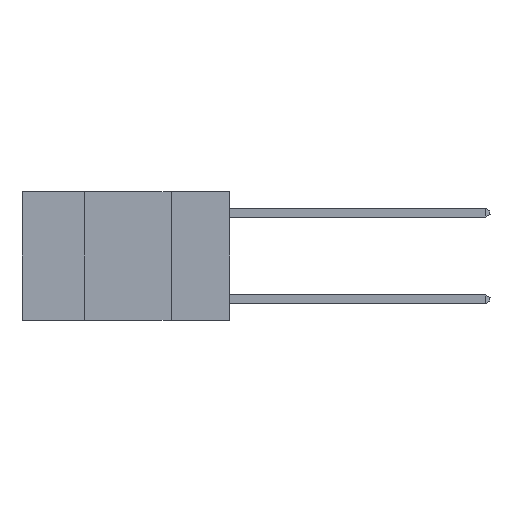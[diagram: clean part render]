
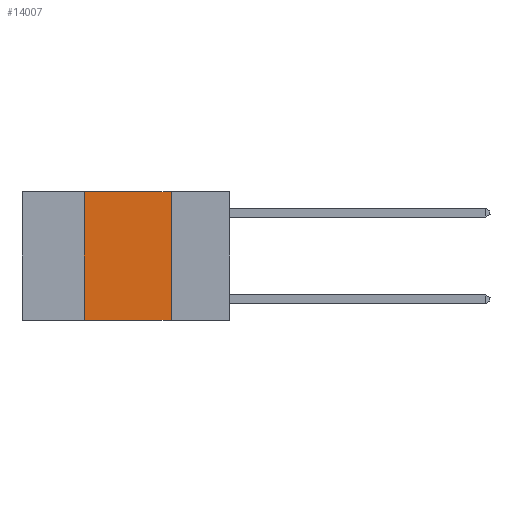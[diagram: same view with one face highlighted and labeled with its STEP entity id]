
A CAD part, left-side view. The second image highlights one B-rep face of the part: STEP entity #14007.
In plain terms, the highlighted planar face has unit normal (-1, 0, 0).
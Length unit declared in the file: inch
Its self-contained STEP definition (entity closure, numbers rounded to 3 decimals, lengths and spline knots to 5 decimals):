
#234 = FACE_OUTER_BOUND ( 'NONE', #3559, .T. ) ;
#333 = CARTESIAN_POINT ( 'NONE',  ( 0., 0.17, 0. ) ) ;
#428 = EDGE_CURVE ( 'NONE', #11161, #1083, #12738, .T. ) ;
#554 = ORIENTED_EDGE ( 'NONE', *, *, #428, .F. ) ;
#1083 = VERTEX_POINT ( 'NONE', #3482 ) ;
#1178 = DIRECTION ( 'NONE',  ( 0., 0., 1. ) ) ;
#1195 = VERTEX_POINT ( 'NONE', #333 ) ;
#1783 = DIRECTION ( 'NONE',  ( 0., -1., 0. ) ) ;
#2016 = VERTEX_POINT ( 'NONE', #6250 ) ;
#2127 = ORIENTED_EDGE ( 'NONE', *, *, #10634, .F. ) ;
#2310 = DIRECTION ( 'NONE',  ( 0., 0., -1. ) ) ;
#2327 = ORIENTED_EDGE ( 'NONE', *, *, #3384, .T. ) ;
#2596 = LINE ( 'NONE', #10588, #4030 ) ;
#3384 = EDGE_CURVE ( 'NONE', #11161, #2016, #12032, .T. ) ;
#3482 = CARTESIAN_POINT ( 'NONE',  ( 0., 0.42, 0. ) ) ;
#3559 = EDGE_LOOP ( 'NONE', ( #2127, #9063, #554, #2327 ) ) ;
#4030 = VECTOR ( 'NONE', #9686, 39.37008 ) ;
#4079 = LINE ( 'NONE', #12203, #8187 ) ;
#5051 = CARTESIAN_POINT ( 'NONE',  ( 0., 0.6, -0.37 ) ) ;
#5824 = CARTESIAN_POINT ( 'NONE',  ( 0., 0.6, 0. ) ) ;
#5971 = DIRECTION ( 'NONE',  ( 1., 0., 0. ) ) ;
#6175 = CARTESIAN_POINT ( 'NONE',  ( 0., 0.42, -0.37 ) ) ;
#6250 = CARTESIAN_POINT ( 'NONE',  ( 0., 0.17, -0.37 ) ) ;
#7342 = DIRECTION ( 'NONE',  ( 0., -1., 0. ) ) ;
#7833 = VECTOR ( 'NONE', #7342, 39.37008 ) ;
#8046 = PLANE ( 'NONE',  #14016 ) ;
#8184 = EDGE_CURVE ( 'NONE', #1083, #1195, #4079, .T. ) ;
#8187 = VECTOR ( 'NONE', #1783, 39.37008 ) ;
#9063 = ORIENTED_EDGE ( 'NONE', *, *, #8184, .F. ) ;
#9686 = DIRECTION ( 'NONE',  ( 0., 0., -1. ) ) ;
#10588 = CARTESIAN_POINT ( 'NONE',  ( 0., 0.17, 0. ) ) ;
#10634 = EDGE_CURVE ( 'NONE', #1195, #2016, #2596, .T. ) ;
#11161 = VERTEX_POINT ( 'NONE', #6175 ) ;
#11613 = CARTESIAN_POINT ( 'NONE',  ( 0., 0.42, 0. ) ) ;
#12032 = LINE ( 'NONE', #5051, #7833 ) ;
#12203 = CARTESIAN_POINT ( 'NONE',  ( 0., 0.6, 0. ) ) ;
#12738 = LINE ( 'NONE', #11613, #13140 ) ;
#13140 = VECTOR ( 'NONE', #1178, 39.37008 ) ;
#14007 = ADVANCED_FACE ( 'NONE', ( #234 ), #8046, .F. ) ;
#14016 = AXIS2_PLACEMENT_3D ( 'NONE', #5824, #5971, #2310 ) ;
